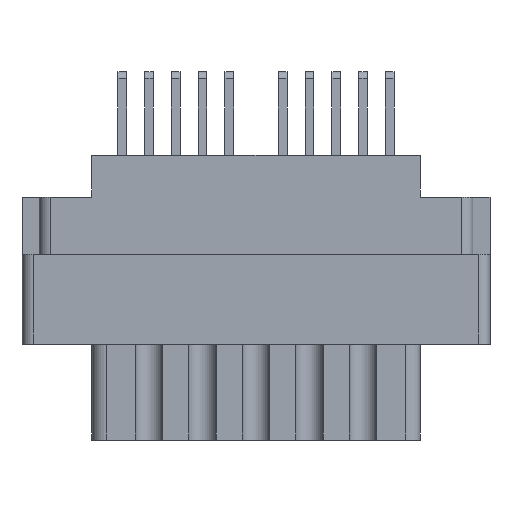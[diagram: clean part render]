
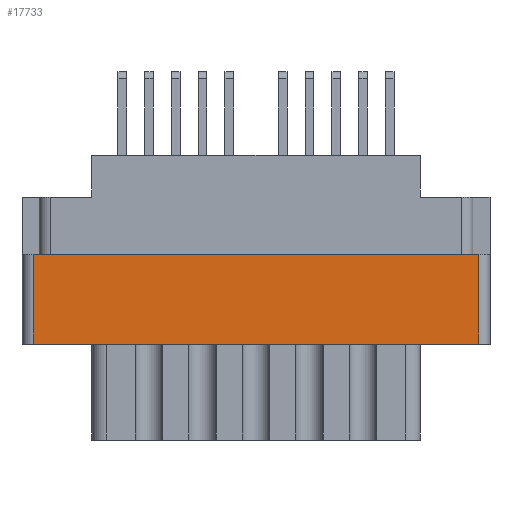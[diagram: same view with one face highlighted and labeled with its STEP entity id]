
A CAD part, front view. The second image highlights one B-rep face of the part: STEP entity #17733.
In plain terms, the highlighted planar face has unit normal (0, -1, 0).
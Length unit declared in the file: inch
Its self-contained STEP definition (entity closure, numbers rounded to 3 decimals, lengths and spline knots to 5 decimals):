
#2591 = CARTESIAN_POINT ( 'NONE',  ( 0.624, -0.343, -0.529 ) ) ;
#3044 = EDGE_LOOP ( 'NONE', ( #5932, #13137, #5088, #6113 ) ) ;
#4008 = DIRECTION ( 'NONE',  ( 0., 0., -1. ) ) ;
#4056 = EDGE_CURVE ( 'NONE', #23854, #17916, #22925, .T. ) ;
#4372 = VECTOR ( 'NONE', #4008, 39.37008 ) ;
#4881 = VERTEX_POINT ( 'NONE', #2591 ) ;
#5088 = ORIENTED_EDGE ( 'NONE', *, *, #17211, .F. ) ;
#5932 = ORIENTED_EDGE ( 'NONE', *, *, #4056, .F. ) ;
#6113 = ORIENTED_EDGE ( 'NONE', *, *, #9131, .T. ) ;
#6381 = CARTESIAN_POINT ( 'NONE',  ( 0., -0.343, -0.277 ) ) ;
#6982 = PLANE ( 'NONE',  #20493 ) ;
#7108 = CARTESIAN_POINT ( 'NONE',  ( -0.656, -0.343, -0.798 ) ) ;
#7392 = CARTESIAN_POINT ( 'NONE',  ( -0.624, -0.343, -0.798 ) ) ;
#7818 = VECTOR ( 'NONE', #21998, 39.37008 ) ;
#8568 = VERTEX_POINT ( 'NONE', #21909 ) ;
#8902 = VECTOR ( 'NONE', #17547, 39.37008 ) ;
#9131 = EDGE_CURVE ( 'NONE', #4881, #17916, #10886, .T. ) ;
#9883 = DIRECTION ( 'NONE',  ( 1., 0., 0. ) ) ;
#10218 = EDGE_CURVE ( 'NONE', #23854, #8568, #20555, .T. ) ;
#10886 = LINE ( 'NONE', #18005, #7818 ) ;
#12393 = CARTESIAN_POINT ( 'NONE',  ( -0.624, -0.343, -0.277 ) ) ;
#12994 = CARTESIAN_POINT ( 'NONE',  ( 0.624, -0.343, -0.277 ) ) ;
#13137 = ORIENTED_EDGE ( 'NONE', *, *, #10218, .T. ) ;
#14469 = DIRECTION ( 'NONE',  ( 0., -1., 0. ) ) ;
#17211 = EDGE_CURVE ( 'NONE', #4881, #8568, #21052, .T. ) ;
#17547 = DIRECTION ( 'NONE',  ( -1., 0., 0. ) ) ;
#17733 = ADVANCED_FACE ( 'NONE', ( #23521 ), #6982, .T. ) ;
#17916 = VERTEX_POINT ( 'NONE', #12994 ) ;
#18005 = CARTESIAN_POINT ( 'NONE',  ( 0.624, -0.343, -0.798 ) ) ;
#20493 = AXIS2_PLACEMENT_3D ( 'NONE', #7108, #14469, #21841 ) ;
#20555 = LINE ( 'NONE', #7392, #4372 ) ;
#21052 = LINE ( 'NONE', #21167, #8902 ) ;
#21167 = CARTESIAN_POINT ( 'NONE',  ( 0., -0.343, -0.529 ) ) ;
#21841 = DIRECTION ( 'NONE',  ( 0., 0., -1. ) ) ;
#21909 = CARTESIAN_POINT ( 'NONE',  ( -0.624, -0.343, -0.529 ) ) ;
#21998 = DIRECTION ( 'NONE',  ( 0., 0., 1. ) ) ;
#22925 = LINE ( 'NONE', #6381, #23830 ) ;
#23521 = FACE_OUTER_BOUND ( 'NONE', #3044, .T. ) ;
#23830 = VECTOR ( 'NONE', #9883, 39.37008 ) ;
#23854 = VERTEX_POINT ( 'NONE', #12393 ) ;
